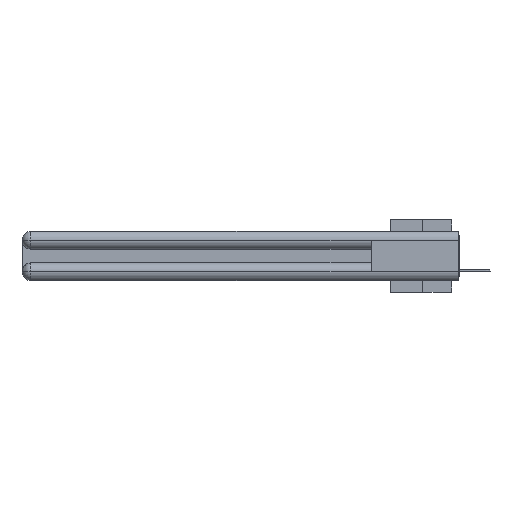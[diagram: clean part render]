
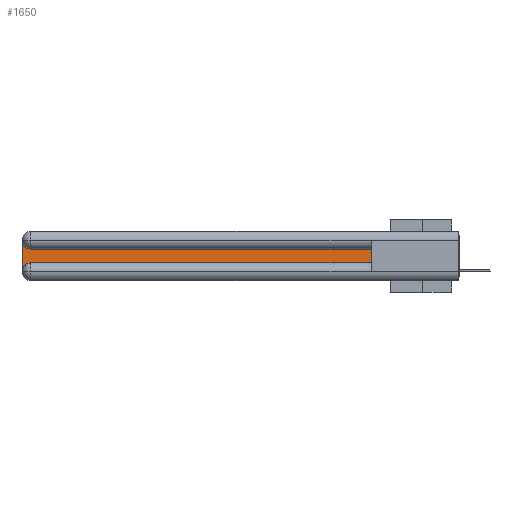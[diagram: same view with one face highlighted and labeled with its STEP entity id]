
A CAD part, left-side view. The second image highlights one B-rep face of the part: STEP entity #1650.
In plain terms, the highlighted planar face has unit normal (-1, 0, 0).
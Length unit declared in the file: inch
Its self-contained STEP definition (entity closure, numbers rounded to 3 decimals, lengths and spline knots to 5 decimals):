
#822 = VERTEX_POINT ( 'NONE', #15763 ) ;
#1391 = VERTEX_POINT ( 'NONE', #11668 ) ;
#1650 = ADVANCED_FACE ( 'NONE', ( #5569 ), #31782, .F. ) ;
#2395 = DIRECTION ( 'NONE',  ( 0., -1., 0. ) ) ;
#2914 = VERTEX_POINT ( 'NONE', #25138 ) ;
#4020 = CARTESIAN_POINT ( 'NONE',  ( 0.075, 2.94, -0.2775 ) ) ;
#4130 = DIRECTION ( 'NONE',  ( 0., 1., 0. ) ) ;
#5047 = EDGE_CURVE ( 'NONE', #1391, #14080, #16294, .T. ) ;
#5569 = FACE_OUTER_BOUND ( 'NONE', #26654, .T. ) ;
#5907 = ORIENTED_EDGE ( 'NONE', *, *, #8236, .T. ) ;
#6082 = CARTESIAN_POINT ( 'NONE',  ( 0.075, 3., -0.2175 ) ) ;
#6222 = VECTOR ( 'NONE', #2395, 39.37008 ) ;
#6648 = AXIS2_PLACEMENT_3D ( 'NONE', #21025, #20859, #10604 ) ;
#7950 = CARTESIAN_POINT ( 'NONE',  ( 0.075, 0.6, -0.2175 ) ) ;
#8236 = EDGE_CURVE ( 'NONE', #11379, #1391, #27078, .T. ) ;
#9651 = DIRECTION ( 'NONE',  ( 0., 0., 1. ) ) ;
#10457 = DIRECTION ( 'NONE',  ( 0., 0., -1. ) ) ;
#10604 = DIRECTION ( 'NONE',  ( 0., 0., -1. ) ) ;
#11181 = VECTOR ( 'NONE', #16666, 39.37008 ) ;
#11376 = DIRECTION ( 'NONE',  ( 0., 0., -1. ) ) ;
#11379 = VERTEX_POINT ( 'NONE', #11907 ) ;
#11668 = CARTESIAN_POINT ( 'NONE',  ( 0.075, 3., -0.2775 ) ) ;
#11907 = CARTESIAN_POINT ( 'NONE',  ( 0.075, 3., -0.0625 ) ) ;
#12977 = EDGE_CURVE ( 'NONE', #14080, #31540, #26171, .T. ) ;
#13060 = CARTESIAN_POINT ( 'NONE',  ( 0.075, 2.94, -0.0625 ) ) ;
#14080 = VERTEX_POINT ( 'NONE', #33668 ) ;
#14112 = CARTESIAN_POINT ( 'NONE',  ( 0.075, 0.6, -0.2175 ) ) ;
#14574 = AXIS2_PLACEMENT_3D ( 'NONE', #13060, #23471, #10457 ) ;
#14844 = LINE ( 'NONE', #22339, #15514 ) ;
#14886 = ORIENTED_EDGE ( 'NONE', *, *, #28277, .T. ) ;
#15514 = VECTOR ( 'NONE', #9651, 39.37008 ) ;
#15763 = CARTESIAN_POINT ( 'NONE',  ( 0.075, 2.94, -0.1225 ) ) ;
#16294 = CIRCLE ( 'NONE', #34056, 0.06 ) ;
#16666 = DIRECTION ( 'NONE',  ( 0., 0., -1. ) ) ;
#19711 = EDGE_CURVE ( 'NONE', #2914, #822, #27907, .T. ) ;
#20859 = DIRECTION ( 'NONE',  ( 1., 0., 0. ) ) ;
#21025 = CARTESIAN_POINT ( 'NONE',  ( 0.075, 3., -0.1225 ) ) ;
#22063 = ORIENTED_EDGE ( 'NONE', *, *, #23389, .T. ) ;
#22339 = CARTESIAN_POINT ( 'NONE',  ( 0.075, 0.6, -0.2175 ) ) ;
#23112 = DIRECTION ( 'NONE',  ( 1., 0., 0. ) ) ;
#23389 = EDGE_CURVE ( 'NONE', #31540, #2914, #14844, .T. ) ;
#23471 = DIRECTION ( 'NONE',  ( 1., 0., 0. ) ) ;
#24024 = CIRCLE ( 'NONE', #14574, 0.06 ) ;
#25035 = ORIENTED_EDGE ( 'NONE', *, *, #12977, .T. ) ;
#25138 = CARTESIAN_POINT ( 'NONE',  ( 0.075, 0.6, -0.1225 ) ) ;
#25653 = CARTESIAN_POINT ( 'NONE',  ( 0.075, 0.6, -0.1225 ) ) ;
#26171 = LINE ( 'NONE', #7950, #6222 ) ;
#26530 = ORIENTED_EDGE ( 'NONE', *, *, #19711, .T. ) ;
#26654 = EDGE_LOOP ( 'NONE', ( #26530, #14886, #5907, #28847, #25035, #22063 ) ) ;
#27078 = LINE ( 'NONE', #6082, #11181 ) ;
#27907 = LINE ( 'NONE', #25653, #28099 ) ;
#28099 = VECTOR ( 'NONE', #4130, 39.37008 ) ;
#28277 = EDGE_CURVE ( 'NONE', #822, #11379, #24024, .T. ) ;
#28847 = ORIENTED_EDGE ( 'NONE', *, *, #5047, .T. ) ;
#31540 = VERTEX_POINT ( 'NONE', #14112 ) ;
#31782 = PLANE ( 'NONE',  #6648 ) ;
#33668 = CARTESIAN_POINT ( 'NONE',  ( 0.075, 2.94, -0.2175 ) ) ;
#34056 = AXIS2_PLACEMENT_3D ( 'NONE', #4020, #23112, #11376 ) ;
